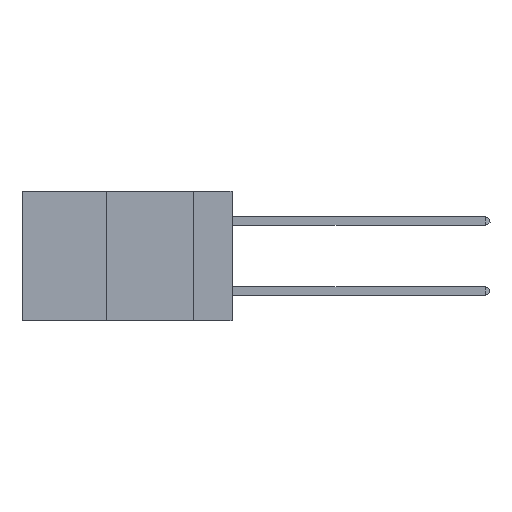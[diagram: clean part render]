
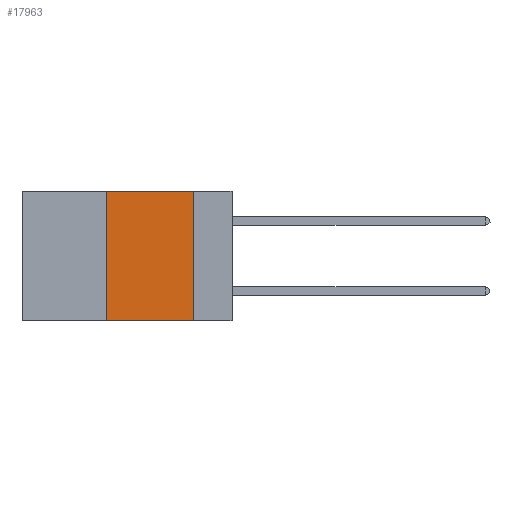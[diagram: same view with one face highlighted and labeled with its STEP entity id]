
A CAD part, left-side view. The second image highlights one B-rep face of the part: STEP entity #17963.
In plain terms, the highlighted planar face has unit normal (-1, 0, 0).
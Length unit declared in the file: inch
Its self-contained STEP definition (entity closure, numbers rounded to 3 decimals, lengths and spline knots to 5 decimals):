
#490 = LINE ( 'NONE', #10581, #7008 ) ;
#616 = CARTESIAN_POINT ( 'NONE',  ( 0., 0.6, 0. ) ) ;
#694 = DIRECTION ( 'NONE',  ( 0., -1., 0. ) ) ;
#2680 = CARTESIAN_POINT ( 'NONE',  ( 0., 0.36, -0.37 ) ) ;
#4051 = EDGE_CURVE ( 'NONE', #18848, #11081, #490, .T. ) ;
#4357 = VECTOR ( 'NONE', #17525, 39.37008 ) ;
#4896 = LINE ( 'NONE', #616, #14016 ) ;
#5951 = DIRECTION ( 'NONE',  ( 0., 0., -1. ) ) ;
#6923 = LINE ( 'NONE', #12282, #4357 ) ;
#7008 = VECTOR ( 'NONE', #23417, 39.37008 ) ;
#7761 = VERTEX_POINT ( 'NONE', #18671 ) ;
#7790 = AXIS2_PLACEMENT_3D ( 'NONE', #16866, #22292, #5951 ) ;
#8702 = CARTESIAN_POINT ( 'NONE',  ( 0., 0.11, -0.37 ) ) ;
#9979 = ORIENTED_EDGE ( 'NONE', *, *, #16112, .F. ) ;
#10175 = ORIENTED_EDGE ( 'NONE', *, *, #4051, .T. ) ;
#10581 = CARTESIAN_POINT ( 'NONE',  ( 0., 0.6, -0.37 ) ) ;
#10933 = CARTESIAN_POINT ( 'NONE',  ( 0., 0.11, 0. ) ) ;
#11081 = VERTEX_POINT ( 'NONE', #8702 ) ;
#11965 = EDGE_LOOP ( 'NONE', ( #20101, #9979, #17182, #10175 ) ) ;
#12282 = CARTESIAN_POINT ( 'NONE',  ( 0., 0.36, 0. ) ) ;
#12474 = CARTESIAN_POINT ( 'NONE',  ( 0., 0.11, 0. ) ) ;
#12766 = DIRECTION ( 'NONE',  ( 0., 0., -1. ) ) ;
#13014 = LINE ( 'NONE', #10933, #23338 ) ;
#13767 = VERTEX_POINT ( 'NONE', #12474 ) ;
#14016 = VECTOR ( 'NONE', #694, 39.37008 ) ;
#14874 = EDGE_CURVE ( 'NONE', #18848, #7761, #6923, .T. ) ;
#16112 = EDGE_CURVE ( 'NONE', #7761, #13767, #4896, .T. ) ;
#16782 = PLANE ( 'NONE',  #7790 ) ;
#16866 = CARTESIAN_POINT ( 'NONE',  ( 0., 0.6, 0. ) ) ;
#17126 = FACE_OUTER_BOUND ( 'NONE', #11965, .T. ) ;
#17182 = ORIENTED_EDGE ( 'NONE', *, *, #14874, .F. ) ;
#17525 = DIRECTION ( 'NONE',  ( 0., 0., 1. ) ) ;
#17963 = ADVANCED_FACE ( 'NONE', ( #17126 ), #16782, .F. ) ;
#18671 = CARTESIAN_POINT ( 'NONE',  ( 0., 0.36, 0. ) ) ;
#18848 = VERTEX_POINT ( 'NONE', #2680 ) ;
#20101 = ORIENTED_EDGE ( 'NONE', *, *, #23191, .F. ) ;
#22292 = DIRECTION ( 'NONE',  ( 1., 0., 0. ) ) ;
#23191 = EDGE_CURVE ( 'NONE', #13767, #11081, #13014, .T. ) ;
#23338 = VECTOR ( 'NONE', #12766, 39.37008 ) ;
#23417 = DIRECTION ( 'NONE',  ( 0., -1., 0. ) ) ;
